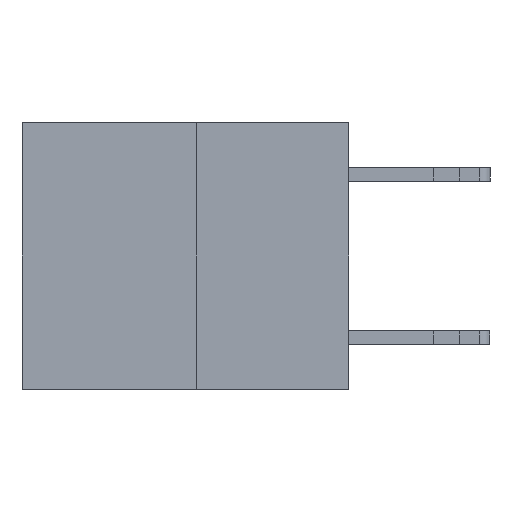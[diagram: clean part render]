
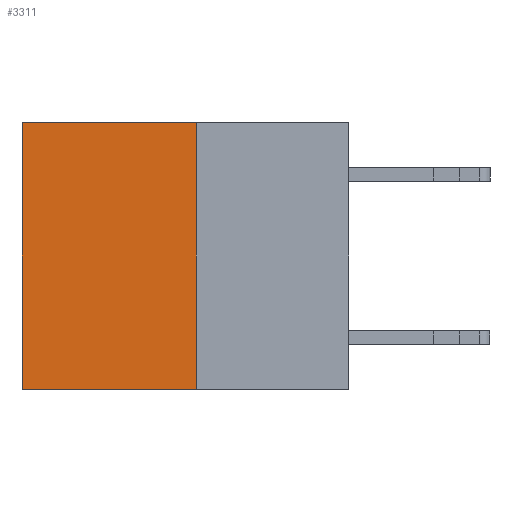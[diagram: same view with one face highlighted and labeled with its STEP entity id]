
A CAD part, left-side view. The second image highlights one B-rep face of the part: STEP entity #3311.
In plain terms, the highlighted planar face has unit normal (-1, 0, 0).
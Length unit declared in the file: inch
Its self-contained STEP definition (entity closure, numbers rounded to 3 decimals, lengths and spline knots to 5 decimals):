
#260 = VECTOR ( 'NONE', #3373, 39.37008 ) ;
#670 = VERTEX_POINT ( 'NONE', #1720 ) ;
#806 = FACE_OUTER_BOUND ( 'NONE', #9212, .T. ) ;
#1173 = VECTOR ( 'NONE', #7493, 39.37008 ) ;
#1714 = AXIS2_PLACEMENT_3D ( 'NONE', #3128, #4326, #8562 ) ;
#1720 = CARTESIAN_POINT ( 'NONE',  ( 0.3165, 0.6, 0. ) ) ;
#1887 = PLANE ( 'NONE',  #1714 ) ;
#1920 = EDGE_CURVE ( 'NONE', #670, #10220, #6285, .T. ) ;
#2237 = CARTESIAN_POINT ( 'NONE',  ( 0.3165, 0.28, -0.49 ) ) ;
#2535 = VECTOR ( 'NONE', #7680, 39.37008 ) ;
#2643 = EDGE_CURVE ( 'NONE', #11791, #670, #8821, .T. ) ;
#3070 = CARTESIAN_POINT ( 'NONE',  ( 0.3165, 0.28, 0. ) ) ;
#3128 = CARTESIAN_POINT ( 'NONE',  ( 0.3165, 0.28, -0.49 ) ) ;
#3311 = ADVANCED_FACE ( 'NONE', ( #806 ), #1887, .F. ) ;
#3373 = DIRECTION ( 'NONE',  ( 0., 1., 0. ) ) ;
#4326 = DIRECTION ( 'NONE',  ( 1., 0., 0. ) ) ;
#4371 = EDGE_CURVE ( 'NONE', #5626, #10220, #10297, .T. ) ;
#5626 = VERTEX_POINT ( 'NONE', #12375 ) ;
#6285 = LINE ( 'NONE', #7735, #2535 ) ;
#6854 = ORIENTED_EDGE ( 'NONE', *, *, #11053, .F. ) ;
#7493 = DIRECTION ( 'NONE',  ( 0., 0., -1. ) ) ;
#7680 = DIRECTION ( 'NONE',  ( 0., 0., -1. ) ) ;
#7696 = ORIENTED_EDGE ( 'NONE', *, *, #4371, .F. ) ;
#7735 = CARTESIAN_POINT ( 'NONE',  ( 0.3165, 0.6, -0.49 ) ) ;
#7972 = CARTESIAN_POINT ( 'NONE',  ( 0.3165, 0.6, -0.49 ) ) ;
#8122 = CARTESIAN_POINT ( 'NONE',  ( 0.3165, 0.28, 0. ) ) ;
#8319 = DIRECTION ( 'NONE',  ( 0., 1., 0. ) ) ;
#8330 = LINE ( 'NONE', #13027, #1173 ) ;
#8562 = DIRECTION ( 'NONE',  ( 0., 0., -1. ) ) ;
#8821 = LINE ( 'NONE', #3070, #12922 ) ;
#9212 = EDGE_LOOP ( 'NONE', ( #13019, #7696, #6854, #13074 ) ) ;
#10220 = VERTEX_POINT ( 'NONE', #7972 ) ;
#10297 = LINE ( 'NONE', #2237, #260 ) ;
#11053 = EDGE_CURVE ( 'NONE', #11791, #5626, #8330, .T. ) ;
#11791 = VERTEX_POINT ( 'NONE', #8122 ) ;
#12375 = CARTESIAN_POINT ( 'NONE',  ( 0.3165, 0.28, -0.49 ) ) ;
#12922 = VECTOR ( 'NONE', #8319, 39.37008 ) ;
#13019 = ORIENTED_EDGE ( 'NONE', *, *, #1920, .T. ) ;
#13027 = CARTESIAN_POINT ( 'NONE',  ( 0.3165, 0.28, -0.49 ) ) ;
#13074 = ORIENTED_EDGE ( 'NONE', *, *, #2643, .T. ) ;
